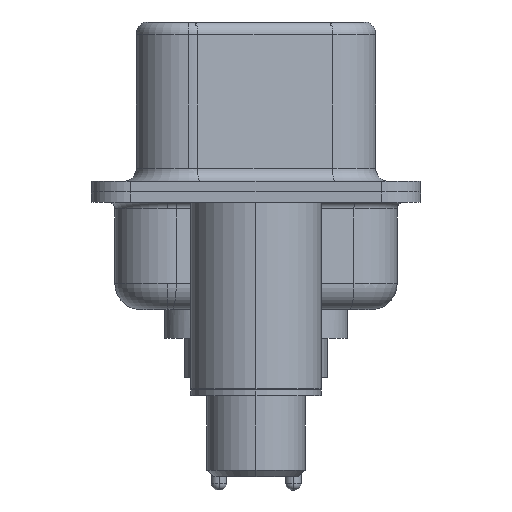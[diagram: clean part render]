
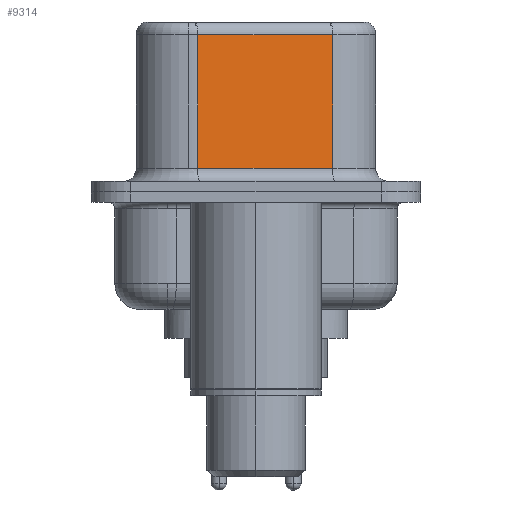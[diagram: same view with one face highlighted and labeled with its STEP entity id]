
A CAD part, left-side view. The second image highlights one B-rep face of the part: STEP entity #9314.
In plain terms, the highlighted planar face has unit normal (-0.985, -0.174, 0).
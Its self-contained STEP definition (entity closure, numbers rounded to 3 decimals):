
#864 = EDGE_CURVE ( 'NONE', #14204, #21509, #18795, .T. ) ;
#1544 = FACE_OUTER_BOUND ( 'NONE', #12323, .T. ) ;
#3648 = LINE ( 'NONE', #15122, #14219 ) ;
#3754 = AXIS2_PLACEMENT_3D ( 'NONE', #18554, #8051, #22791 ) ;
#4611 = EDGE_CURVE ( 'NONE', #14204, #14584, #20576, .T. ) ;
#5494 = CARTESIAN_POINT ( 'NONE',  ( 3.67, 2.233, 0.9 ) ) ;
#5919 = PLANE ( 'NONE',  #3754 ) ;
#6601 = DIRECTION ( 'NONE',  ( 0., 0., -1. ) ) ;
#8051 = DIRECTION ( 'NONE',  ( 0.985, 0.174, 0. ) ) ;
#9314 = ADVANCED_FACE ( 'NONE', ( #1544 ), #5919, .F. ) ;
#10692 = VECTOR ( 'NONE', #11278, 1000. ) ;
#11101 = CARTESIAN_POINT ( 'NONE',  ( 4.58, -2.927, 6.52 ) ) ;
#11278 = DIRECTION ( 'NONE',  ( 0., 0., -1. ) ) ;
#12323 = EDGE_LOOP ( 'NONE', ( #14406, #27163, #17357, #12941 ) ) ;
#12941 = ORIENTED_EDGE ( 'NONE', *, *, #25871, .T. ) ;
#14204 = VERTEX_POINT ( 'NONE', #23974 ) ;
#14219 = VECTOR ( 'NONE', #21494, 1000. ) ;
#14406 = ORIENTED_EDGE ( 'NONE', *, *, #4611, .F. ) ;
#14575 = EDGE_CURVE ( 'NONE', #21509, #15559, #21950, .T. ) ;
#14584 = VERTEX_POINT ( 'NONE', #25631 ) ;
#15122 = CARTESIAN_POINT ( 'NONE',  ( 4.58, -2.927, 0.9 ) ) ;
#15559 = VERTEX_POINT ( 'NONE', #5494 ) ;
#17357 = ORIENTED_EDGE ( 'NONE', *, *, #14575, .T. ) ;
#18554 = CARTESIAN_POINT ( 'NONE',  ( 4.58, -2.927, 6.52 ) ) ;
#18795 = LINE ( 'NONE', #22515, #23084 ) ;
#19222 = CARTESIAN_POINT ( 'NONE',  ( 3.67, 2.233, 6.52 ) ) ;
#20576 = LINE ( 'NONE', #11101, #10692 ) ;
#21494 = DIRECTION ( 'NONE',  ( 0.174, -0.985, 0. ) ) ;
#21509 = VERTEX_POINT ( 'NONE', #27216 ) ;
#21950 = LINE ( 'NONE', #19222, #26958 ) ;
#22515 = CARTESIAN_POINT ( 'NONE',  ( 4.58, -2.927, 6.02 ) ) ;
#22791 = DIRECTION ( 'NONE',  ( -0.174, 0.985, 0. ) ) ;
#23084 = VECTOR ( 'NONE', #24531, 1000. ) ;
#23974 = CARTESIAN_POINT ( 'NONE',  ( 4.58, -2.927, 6.02 ) ) ;
#24531 = DIRECTION ( 'NONE',  ( -0.174, 0.985, 0. ) ) ;
#25631 = CARTESIAN_POINT ( 'NONE',  ( 4.58, -2.927, 0.9 ) ) ;
#25871 = EDGE_CURVE ( 'NONE', #15559, #14584, #3648, .T. ) ;
#26958 = VECTOR ( 'NONE', #6601, 1000. ) ;
#27163 = ORIENTED_EDGE ( 'NONE', *, *, #864, .T. ) ;
#27216 = CARTESIAN_POINT ( 'NONE',  ( 3.67, 2.233, 6.02 ) ) ;
